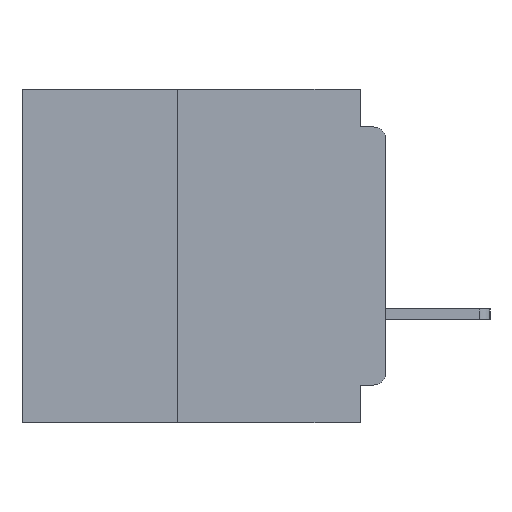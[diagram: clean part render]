
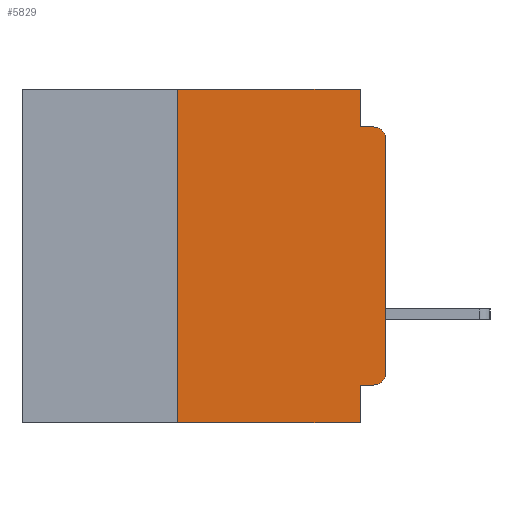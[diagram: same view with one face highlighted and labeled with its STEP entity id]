
A CAD part, left-side view. The second image highlights one B-rep face of the part: STEP entity #5829.
In plain terms, the highlighted planar face has unit normal (-1, 0, 0).
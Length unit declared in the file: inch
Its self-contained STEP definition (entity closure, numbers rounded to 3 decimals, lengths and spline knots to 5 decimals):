
#14 = ORIENTED_EDGE ( 'NONE', *, *, #32102, .F. ) ;
#115 = LINE ( 'NONE', #43882, #38112 ) ;
#262 = LINE ( 'NONE', #15898, #39388 ) ;
#682 = EDGE_CURVE ( 'NONE', #19157, #6265, #47262, .T. ) ;
#770 = CIRCLE ( 'NONE', #9754, 0.015 ) ;
#1088 = CARTESIAN_POINT ( 'NONE',  ( 0., 0.015, -0.355 ) ) ;
#1220 = CARTESIAN_POINT ( 'NONE',  ( 0., 0.437, -0.4 ) ) ;
#1560 = ORIENTED_EDGE ( 'NONE', *, *, #46874, .F. ) ;
#1604 = VERTEX_POINT ( 'NONE', #21677 ) ;
#1832 = VERTEX_POINT ( 'NONE', #8187 ) ;
#2092 = ORIENTED_EDGE ( 'NONE', *, *, #5168, .F. ) ;
#5168 = EDGE_CURVE ( 'NONE', #1832, #43164, #40159, .T. ) ;
#5399 = DIRECTION ( 'NONE',  ( 0., 0., -1. ) ) ;
#5822 = CARTESIAN_POINT ( 'NONE',  ( 0., 0.437, 0. ) ) ;
#5829 = ADVANCED_FACE ( 'NONE', ( #30948 ), #16830, .F. ) ;
#5853 = CARTESIAN_POINT ( 'NONE',  ( 0., 0.031, 0. ) ) ;
#6090 = EDGE_LOOP ( 'NONE', ( #36993, #37839, #23849, #20249, #2092, #14, #45967, #11535, #1560, #13673 ) ) ;
#6265 = VERTEX_POINT ( 'NONE', #45006 ) ;
#7686 = AXIS2_PLACEMENT_3D ( 'NONE', #5822, #13294, #38902 ) ;
#8187 = CARTESIAN_POINT ( 'NONE',  ( 0., 0.25, 0. ) ) ;
#8569 = CARTESIAN_POINT ( 'NONE',  ( 0., 0., -0.045 ) ) ;
#8733 = DIRECTION ( 'NONE',  ( 0., -1., 0. ) ) ;
#9140 = CARTESIAN_POINT ( 'NONE',  ( 0., 0.437, 0. ) ) ;
#9754 = AXIS2_PLACEMENT_3D ( 'NONE', #42616, #20751, #46228 ) ;
#10474 = DIRECTION ( 'NONE',  ( -1., 0., 0. ) ) ;
#10961 = VECTOR ( 'NONE', #12860, 39.37008 ) ;
#11535 = ORIENTED_EDGE ( 'NONE', *, *, #15781, .F. ) ;
#12067 = VERTEX_POINT ( 'NONE', #34062 ) ;
#12207 = VECTOR ( 'NONE', #31383, 39.37008 ) ;
#12860 = DIRECTION ( 'NONE',  ( 0., -1., 0. ) ) ;
#12988 = EDGE_CURVE ( 'NONE', #43164, #19157, #13804, .T. ) ;
#13294 = DIRECTION ( 'NONE',  ( 1., 0., 0. ) ) ;
#13673 = ORIENTED_EDGE ( 'NONE', *, *, #22262, .T. ) ;
#13804 = LINE ( 'NONE', #40382, #32123 ) ;
#15291 = AXIS2_PLACEMENT_3D ( 'NONE', #32413, #10474, #36099 ) ;
#15754 = VECTOR ( 'NONE', #5399, 39.37008 ) ;
#15781 = EDGE_CURVE ( 'NONE', #1604, #37873, #25483, .T. ) ;
#15898 = CARTESIAN_POINT ( 'NONE',  ( 0., 0.25, -0.4 ) ) ;
#16830 = PLANE ( 'NONE',  #7686 ) ;
#17593 = CARTESIAN_POINT ( 'NONE',  ( 0., 0.031, -0.045 ) ) ;
#17767 = VERTEX_POINT ( 'NONE', #42618 ) ;
#18230 = VECTOR ( 'NONE', #8733, 39.37008 ) ;
#19157 = VERTEX_POINT ( 'NONE', #17593 ) ;
#20249 = ORIENTED_EDGE ( 'NONE', *, *, #12988, .F. ) ;
#20356 = CIRCLE ( 'NONE', #15291, 0.015 ) ;
#20751 = DIRECTION ( 'NONE',  ( -1., 0., 0. ) ) ;
#21677 = CARTESIAN_POINT ( 'NONE',  ( 0., 0.031, -0.355 ) ) ;
#21950 = LINE ( 'NONE', #27703, #12207 ) ;
#22028 = DIRECTION ( 'NONE',  ( 0., 0., 1. ) ) ;
#22262 = EDGE_CURVE ( 'NONE', #32748, #31776, #770, .T. ) ;
#22889 = EDGE_CURVE ( 'NONE', #31776, #12067, #115, .T. ) ;
#23227 = VECTOR ( 'NONE', #23329, 39.37008 ) ;
#23329 = DIRECTION ( 'NONE',  ( 0., -1., 0. ) ) ;
#23849 = ORIENTED_EDGE ( 'NONE', *, *, #682, .F. ) ;
#25483 = LINE ( 'NONE', #31129, #15754 ) ;
#25695 = DIRECTION ( 'NONE',  ( 0., 0., -1. ) ) ;
#27703 = CARTESIAN_POINT ( 'NONE',  ( 0., 0., -0.355 ) ) ;
#27760 = CARTESIAN_POINT ( 'NONE',  ( 0., 0., -0.34 ) ) ;
#30948 = FACE_OUTER_BOUND ( 'NONE', #6090, .T. ) ;
#31129 = CARTESIAN_POINT ( 'NONE',  ( 0., 0.031, -0.4 ) ) ;
#31383 = DIRECTION ( 'NONE',  ( 0., 1., 0. ) ) ;
#31776 = VERTEX_POINT ( 'NONE', #27760 ) ;
#32102 = EDGE_CURVE ( 'NONE', #17767, #1832, #262, .T. ) ;
#32123 = VECTOR ( 'NONE', #25695, 39.37008 ) ;
#32413 = CARTESIAN_POINT ( 'NONE',  ( 0., 0.015, -0.06 ) ) ;
#32748 = VERTEX_POINT ( 'NONE', #1088 ) ;
#34062 = CARTESIAN_POINT ( 'NONE',  ( 0., 0., -0.06 ) ) ;
#35796 = CARTESIAN_POINT ( 'NONE',  ( 0., 0.031, -0.4 ) ) ;
#36099 = DIRECTION ( 'NONE',  ( 0., 0., -1. ) ) ;
#36993 = ORIENTED_EDGE ( 'NONE', *, *, #22889, .T. ) ;
#37839 = ORIENTED_EDGE ( 'NONE', *, *, #45910, .T. ) ;
#37873 = VERTEX_POINT ( 'NONE', #35796 ) ;
#38112 = VECTOR ( 'NONE', #22028, 39.37008 ) ;
#38902 = DIRECTION ( 'NONE',  ( 0., 0., -1. ) ) ;
#39388 = VECTOR ( 'NONE', #41453, 39.37008 ) ;
#40159 = LINE ( 'NONE', #9140, #10961 ) ;
#40382 = CARTESIAN_POINT ( 'NONE',  ( 0., 0.031, 0. ) ) ;
#41453 = DIRECTION ( 'NONE',  ( 0., 0., 1. ) ) ;
#41505 = LINE ( 'NONE', #1220, #23227 ) ;
#42616 = CARTESIAN_POINT ( 'NONE',  ( 0., 0.015, -0.34 ) ) ;
#42618 = CARTESIAN_POINT ( 'NONE',  ( 0., 0.25, -0.4 ) ) ;
#43164 = VERTEX_POINT ( 'NONE', #5853 ) ;
#43882 = CARTESIAN_POINT ( 'NONE',  ( 0., 0., 0. ) ) ;
#45006 = CARTESIAN_POINT ( 'NONE',  ( 0., 0.015, -0.045 ) ) ;
#45595 = EDGE_CURVE ( 'NONE', #17767, #37873, #41505, .T. ) ;
#45910 = EDGE_CURVE ( 'NONE', #12067, #6265, #20356, .T. ) ;
#45967 = ORIENTED_EDGE ( 'NONE', *, *, #45595, .T. ) ;
#46228 = DIRECTION ( 'NONE',  ( 0., 0., -1. ) ) ;
#46874 = EDGE_CURVE ( 'NONE', #32748, #1604, #21950, .T. ) ;
#47262 = LINE ( 'NONE', #8569, #18230 ) ;
